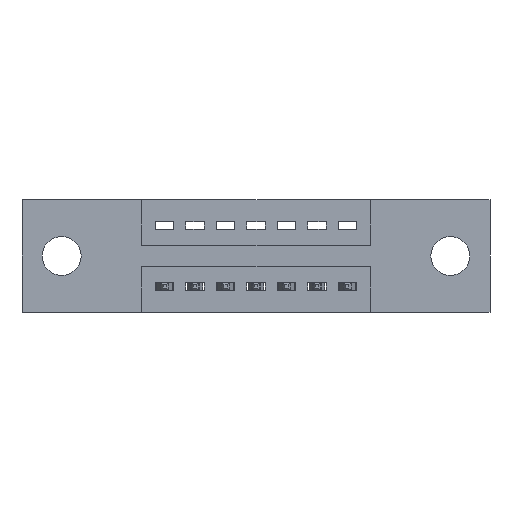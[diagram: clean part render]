
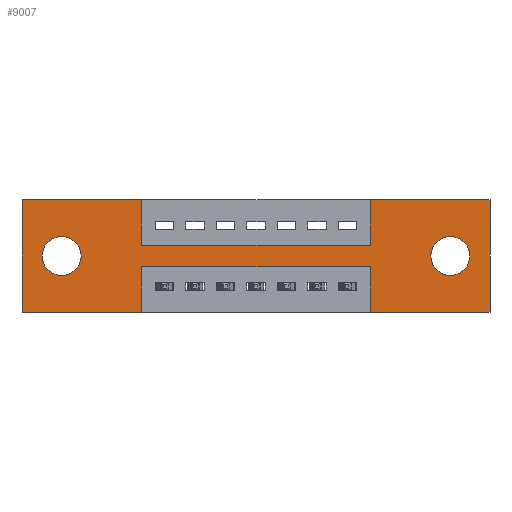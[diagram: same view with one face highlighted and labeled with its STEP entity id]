
A CAD part, front view. The second image highlights one B-rep face of the part: STEP entity #9007.
In plain terms, the highlighted planar face has unit normal (0, -1, 0).
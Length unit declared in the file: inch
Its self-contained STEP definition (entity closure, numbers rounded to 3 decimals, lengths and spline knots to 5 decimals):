
#25 = DIRECTION ( 'NONE',  ( 0., 0., 1. ) ) ;
#50 = CARTESIAN_POINT ( 'NONE',  ( 0.13, 0., -0.185 ) ) ;
#93 = ORIENTED_EDGE ( 'NONE', *, *, #2122, .F. ) ;
#254 = CARTESIAN_POINT ( 'NONE',  ( 0., 0., 0. ) ) ;
#261 = LINE ( 'NONE', #7271, #4995 ) ;
#265 = VECTOR ( 'NONE', #2673, 39.37008 ) ;
#291 = FACE_OUTER_BOUND ( 'NONE', #8696, .T. ) ;
#398 = EDGE_CURVE ( 'NONE', #6932, #7534, #4185, .T. ) ;
#639 = EDGE_CURVE ( 'NONE', #7534, #7404, #665, .T. ) ;
#665 = LINE ( 'NONE', #5649, #7850 ) ;
#694 = AXIS2_PLACEMENT_3D ( 'NONE', #50, #9465, #3227 ) ;
#744 = CARTESIAN_POINT ( 'NONE',  ( 1.1425, 0., -0.22 ) ) ;
#772 = CARTESIAN_POINT ( 'NONE',  ( 1.535, 0., -0.37 ) ) ;
#931 = VERTEX_POINT ( 'NONE', #5070 ) ;
#977 = LINE ( 'NONE', #4579, #5716 ) ;
#997 = VERTEX_POINT ( 'NONE', #7728 ) ;
#1034 = VECTOR ( 'NONE', #5243, 39.37008 ) ;
#1057 = VECTOR ( 'NONE', #1290, 39.37008 ) ;
#1129 = ORIENTED_EDGE ( 'NONE', *, *, #398, .F. ) ;
#1280 = ORIENTED_EDGE ( 'NONE', *, *, #7823, .F. ) ;
#1290 = DIRECTION ( 'NONE',  ( 0., 0., 1. ) ) ;
#1376 = VERTEX_POINT ( 'NONE', #4102 ) ;
#1611 = CARTESIAN_POINT ( 'NONE',  ( 1.405, 0., -0.121 ) ) ;
#1713 = ORIENTED_EDGE ( 'NONE', *, *, #3289, .T. ) ;
#1934 = CARTESIAN_POINT ( 'NONE',  ( 0.3925, 0., -0.37 ) ) ;
#1983 = EDGE_CURVE ( 'NONE', #1376, #7980, #8754, .T. ) ;
#2122 = EDGE_CURVE ( 'NONE', #6070, #3632, #5011, .T. ) ;
#2190 = CARTESIAN_POINT ( 'NONE',  ( 1.1425, 0., -0.15 ) ) ;
#2208 = LINE ( 'NONE', #6580, #4866 ) ;
#2537 = ORIENTED_EDGE ( 'NONE', *, *, #4785, .F. ) ;
#2673 = DIRECTION ( 'NONE',  ( 0., 0., -1. ) ) ;
#2769 = ORIENTED_EDGE ( 'NONE', *, *, #5208, .F. ) ;
#2879 = CARTESIAN_POINT ( 'NONE',  ( 0.3925, 0., -0.22 ) ) ;
#2886 = ORIENTED_EDGE ( 'NONE', *, *, #639, .F. ) ;
#3015 = DIRECTION ( 'NONE',  ( 0., 1., 0. ) ) ;
#3036 = ORIENTED_EDGE ( 'NONE', *, *, #1983, .T. ) ;
#3108 = FACE_BOUND ( 'NONE', #5336, .T. ) ;
#3134 = LINE ( 'NONE', #5625, #5302 ) ;
#3145 = VERTEX_POINT ( 'NONE', #9639 ) ;
#3227 = DIRECTION ( 'NONE',  ( 0., 0., 1. ) ) ;
#3237 = EDGE_CURVE ( 'NONE', #5329, #931, #2208, .T. ) ;
#3289 = EDGE_CURVE ( 'NONE', #7426, #6682, #6440, .T. ) ;
#3315 = CARTESIAN_POINT ( 'NONE',  ( 0., 0., 0. ) ) ;
#3318 = ORIENTED_EDGE ( 'NONE', *, *, #8058, .F. ) ;
#3416 = EDGE_CURVE ( 'NONE', #6682, #7426, #8974, .T. ) ;
#3471 = CARTESIAN_POINT ( 'NONE',  ( 0.3925, 0., -0.22 ) ) ;
#3519 = LINE ( 'NONE', #6704, #8722 ) ;
#3632 = VERTEX_POINT ( 'NONE', #9921 ) ;
#3666 = AXIS2_PLACEMENT_3D ( 'NONE', #4164, #4104, #4043 ) ;
#3740 = ORIENTED_EDGE ( 'NONE', *, *, #3416, .T. ) ;
#3923 = EDGE_CURVE ( 'NONE', #997, #5329, #8152, .T. ) ;
#4043 = DIRECTION ( 'NONE',  ( 0., 0., -1. ) ) ;
#4102 = CARTESIAN_POINT ( 'NONE',  ( 0.13, 0., -0.121 ) ) ;
#4104 = DIRECTION ( 'NONE',  ( 0., -1., 0. ) ) ;
#4164 = CARTESIAN_POINT ( 'NONE',  ( 0., 0., -0.37 ) ) ;
#4185 = LINE ( 'NONE', #3471, #7009 ) ;
#4269 = CARTESIAN_POINT ( 'NONE',  ( 1.405, 0., -0.249 ) ) ;
#4403 = EDGE_CURVE ( 'NONE', #7404, #9477, #261, .T. ) ;
#4522 = CARTESIAN_POINT ( 'NONE',  ( 0.3925, 0., -0.15 ) ) ;
#4579 = CARTESIAN_POINT ( 'NONE',  ( 0., 0., 0. ) ) ;
#4713 = CARTESIAN_POINT ( 'NONE',  ( 0., 0., 0. ) ) ;
#4785 = EDGE_CURVE ( 'NONE', #5434, #3145, #977, .T. ) ;
#4835 = DIRECTION ( 'NONE',  ( 0., 0., -1. ) ) ;
#4866 = VECTOR ( 'NONE', #8256, 39.37008 ) ;
#4995 = VECTOR ( 'NONE', #9421, 39.37008 ) ;
#5011 = LINE ( 'NONE', #9619, #9241 ) ;
#5070 = CARTESIAN_POINT ( 'NONE',  ( 1.1425, 0., -0.37 ) ) ;
#5208 = EDGE_CURVE ( 'NONE', #931, #6932, #3519, .T. ) ;
#5243 = DIRECTION ( 'NONE',  ( 1., 0., 0. ) ) ;
#5263 = DIRECTION ( 'NONE',  ( 0., 0., -1. ) ) ;
#5302 = VECTOR ( 'NONE', #6397, 39.37008 ) ;
#5329 = VERTEX_POINT ( 'NONE', #772 ) ;
#5336 = EDGE_LOOP ( 'NONE', ( #3036, #7163 ) ) ;
#5360 = CARTESIAN_POINT ( 'NONE',  ( 0.13, 0., -0.185 ) ) ;
#5434 = VERTEX_POINT ( 'NONE', #3315 ) ;
#5625 = CARTESIAN_POINT ( 'NONE',  ( 0.3925, 0., 0. ) ) ;
#5649 = CARTESIAN_POINT ( 'NONE',  ( 0.3925, 0., -0.37 ) ) ;
#5716 = VECTOR ( 'NONE', #9965, 39.37008 ) ;
#5747 = DIRECTION ( 'NONE',  ( 0., 0., 1. ) ) ;
#5801 = LINE ( 'NONE', #4713, #1057 ) ;
#5865 = AXIS2_PLACEMENT_3D ( 'NONE', #5360, #3015, #25 ) ;
#5897 = ORIENTED_EDGE ( 'NONE', *, *, #3237, .F. ) ;
#6052 = CARTESIAN_POINT ( 'NONE',  ( 0., 0., -0.37 ) ) ;
#6070 = VERTEX_POINT ( 'NONE', #2190 ) ;
#6277 = VECTOR ( 'NONE', #8816, 39.37008 ) ;
#6387 = LINE ( 'NONE', #4522, #1034 ) ;
#6397 = DIRECTION ( 'NONE',  ( 0., 0., -1. ) ) ;
#6440 = CIRCLE ( 'NONE', #8430, 0.064 ) ;
#6580 = CARTESIAN_POINT ( 'NONE',  ( 0., 0., -0.37 ) ) ;
#6682 = VERTEX_POINT ( 'NONE', #1611 ) ;
#6704 = CARTESIAN_POINT ( 'NONE',  ( 1.1425, 0., -0.37 ) ) ;
#6751 = EDGE_CURVE ( 'NONE', #9477, #5434, #5801, .T. ) ;
#6757 = CIRCLE ( 'NONE', #5865, 0.064 ) ;
#6903 = DIRECTION ( 'NONE',  ( 0., 0., -1. ) ) ;
#6932 = VERTEX_POINT ( 'NONE', #744 ) ;
#7009 = VECTOR ( 'NONE', #7378, 39.37008 ) ;
#7163 = ORIENTED_EDGE ( 'NONE', *, *, #7625, .T. ) ;
#7271 = CARTESIAN_POINT ( 'NONE',  ( 0., 0., -0.37 ) ) ;
#7337 = CARTESIAN_POINT ( 'NONE',  ( 1.535, 0., 0. ) ) ;
#7376 = ORIENTED_EDGE ( 'NONE', *, *, #6751, .F. ) ;
#7378 = DIRECTION ( 'NONE',  ( -1., 0., 0. ) ) ;
#7404 = VERTEX_POINT ( 'NONE', #1934 ) ;
#7426 = VERTEX_POINT ( 'NONE', #4269 ) ;
#7430 = ORIENTED_EDGE ( 'NONE', *, *, #7764, .F. ) ;
#7534 = VERTEX_POINT ( 'NONE', #2879 ) ;
#7574 = CARTESIAN_POINT ( 'NONE',  ( 1.405, 0., -0.185 ) ) ;
#7625 = EDGE_CURVE ( 'NONE', #7980, #1376, #6757, .T. ) ;
#7728 = CARTESIAN_POINT ( 'NONE',  ( 1.535, 0., 0. ) ) ;
#7756 = CARTESIAN_POINT ( 'NONE',  ( 1.405, 0., -0.185 ) ) ;
#7764 = EDGE_CURVE ( 'NONE', #3145, #9896, #3134, .T. ) ;
#7823 = EDGE_CURVE ( 'NONE', #3632, #997, #9299, .T. ) ;
#7850 = VECTOR ( 'NONE', #4835, 39.37008 ) ;
#7980 = VERTEX_POINT ( 'NONE', #8386 ) ;
#8058 = EDGE_CURVE ( 'NONE', #9896, #6070, #6387, .T. ) ;
#8062 = FACE_BOUND ( 'NONE', #8617, .T. ) ;
#8152 = LINE ( 'NONE', #7337, #265 ) ;
#8256 = DIRECTION ( 'NONE',  ( -1., 0., 0. ) ) ;
#8386 = CARTESIAN_POINT ( 'NONE',  ( 0.13, 0., -0.249 ) ) ;
#8430 = AXIS2_PLACEMENT_3D ( 'NONE', #7574, #9867, #5263 ) ;
#8511 = DIRECTION ( 'NONE',  ( 0., 1., 0. ) ) ;
#8568 = AXIS2_PLACEMENT_3D ( 'NONE', #7756, #8511, #6903 ) ;
#8617 = EDGE_LOOP ( 'NONE', ( #3740, #1713 ) ) ;
#8640 = CARTESIAN_POINT ( 'NONE',  ( 0.3925, 0., -0.15 ) ) ;
#8696 = EDGE_LOOP ( 'NONE', ( #2886, #1129, #2769, #5897, #9334, #1280, #93, #3318, #7430, #2537, #7376, #9665 ) ) ;
#8722 = VECTOR ( 'NONE', #9786, 39.37008 ) ;
#8754 = CIRCLE ( 'NONE', #694, 0.064 ) ;
#8799 = PLANE ( 'NONE',  #3666 ) ;
#8816 = DIRECTION ( 'NONE',  ( 1., 0., 0. ) ) ;
#8974 = CIRCLE ( 'NONE', #8568, 0.064 ) ;
#9007 = ADVANCED_FACE ( 'NONE', ( #8062, #3108, #291 ), #8799, .T. ) ;
#9241 = VECTOR ( 'NONE', #5747, 39.37008 ) ;
#9299 = LINE ( 'NONE', #254, #6277 ) ;
#9334 = ORIENTED_EDGE ( 'NONE', *, *, #3923, .F. ) ;
#9421 = DIRECTION ( 'NONE',  ( -1., 0., 0. ) ) ;
#9465 = DIRECTION ( 'NONE',  ( 0., 1., 0. ) ) ;
#9477 = VERTEX_POINT ( 'NONE', #6052 ) ;
#9619 = CARTESIAN_POINT ( 'NONE',  ( 1.1425, 0., 0. ) ) ;
#9639 = CARTESIAN_POINT ( 'NONE',  ( 0.3925, 0., 0. ) ) ;
#9665 = ORIENTED_EDGE ( 'NONE', *, *, #4403, .F. ) ;
#9786 = DIRECTION ( 'NONE',  ( 0., 0., 1. ) ) ;
#9867 = DIRECTION ( 'NONE',  ( 0., 1., 0. ) ) ;
#9896 = VERTEX_POINT ( 'NONE', #8640 ) ;
#9921 = CARTESIAN_POINT ( 'NONE',  ( 1.1425, 0., 0. ) ) ;
#9965 = DIRECTION ( 'NONE',  ( 1., 0., 0. ) ) ;
